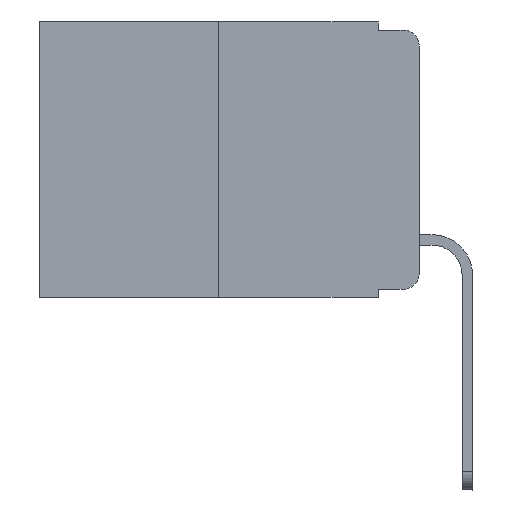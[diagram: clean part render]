
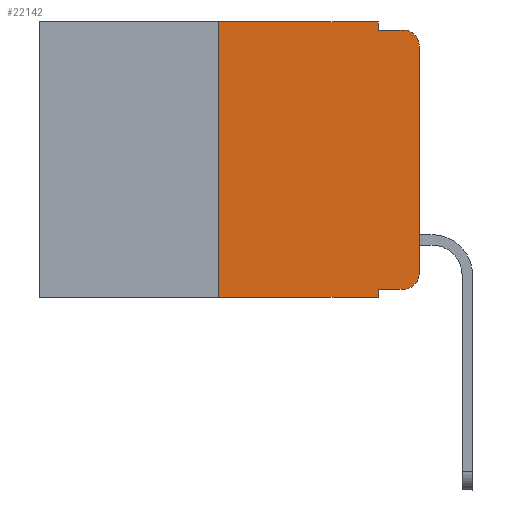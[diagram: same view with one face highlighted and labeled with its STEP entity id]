
A CAD part, left-side view. The second image highlights one B-rep face of the part: STEP entity #22142.
In plain terms, the highlighted planar face has unit normal (-1, 0, 0).
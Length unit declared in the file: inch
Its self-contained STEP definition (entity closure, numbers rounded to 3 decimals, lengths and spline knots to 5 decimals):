
#168 = CARTESIAN_POINT ( 'NONE',  ( 0., 0., -0.313 ) ) ;
#198 = AXIS2_PLACEMENT_3D ( 'NONE', #2361, #24579, #8092 ) ;
#484 = CARTESIAN_POINT ( 'NONE',  ( 0., 0.051, -0.333 ) ) ;
#729 = VERTEX_POINT ( 'NONE', #14420 ) ;
#969 = ORIENTED_EDGE ( 'NONE', *, *, #9742, .T. ) ;
#1007 = LINE ( 'NONE', #8992, #19425 ) ;
#1231 = ORIENTED_EDGE ( 'NONE', *, *, #5311, .F. ) ;
#1653 = ORIENTED_EDGE ( 'NONE', *, *, #17174, .T. ) ;
#1742 = VERTEX_POINT ( 'NONE', #16167 ) ;
#2361 = CARTESIAN_POINT ( 'NONE',  ( 0., 0.02, -0.313 ) ) ;
#2617 = CARTESIAN_POINT ( 'NONE',  ( 0., 0.051, -0.01 ) ) ;
#3530 = CIRCLE ( 'NONE', #18398, 0.02 ) ;
#4014 = ORIENTED_EDGE ( 'NONE', *, *, #21274, .T. ) ;
#4030 = VERTEX_POINT ( 'NONE', #25972 ) ;
#4064 = DIRECTION ( 'NONE',  ( 1., 0., 0. ) ) ;
#4197 = FACE_OUTER_BOUND ( 'NONE', #15719, .T. ) ;
#4251 = VECTOR ( 'NONE', #5102, 39.37008 ) ;
#4290 = CARTESIAN_POINT ( 'NONE',  ( 0., 0.051, -0.333 ) ) ;
#4585 = LINE ( 'NONE', #10703, #9799 ) ;
#4609 = ORIENTED_EDGE ( 'NONE', *, *, #16207, .F. ) ;
#4697 = CARTESIAN_POINT ( 'NONE',  ( 0., 0.02, -0.333 ) ) ;
#5102 = DIRECTION ( 'NONE',  ( 0., 0., 1. ) ) ;
#5311 = EDGE_CURVE ( 'NONE', #1742, #9038, #1007, .T. ) ;
#5446 = LINE ( 'NONE', #19281, #6911 ) ;
#5981 = DIRECTION ( 'NONE',  ( 0., -1., 0. ) ) ;
#6183 = ORIENTED_EDGE ( 'NONE', *, *, #16247, .T. ) ;
#6246 = CARTESIAN_POINT ( 'NONE',  ( 0., 0.02, -0.03 ) ) ;
#6911 = VECTOR ( 'NONE', #5981, 39.37008 ) ;
#7539 = CARTESIAN_POINT ( 'NONE',  ( 0., 0.051, 0. ) ) ;
#8092 = DIRECTION ( 'NONE',  ( 0., 0., -1. ) ) ;
#8992 = CARTESIAN_POINT ( 'NONE',  ( 0., 0.473, 0. ) ) ;
#9038 = VERTEX_POINT ( 'NONE', #22560 ) ;
#9157 = VERTEX_POINT ( 'NONE', #2617 ) ;
#9742 = EDGE_CURVE ( 'NONE', #16116, #15303, #23452, .T. ) ;
#9799 = VECTOR ( 'NONE', #18819, 39.37008 ) ;
#10115 = DIRECTION ( 'NONE',  ( 0., 0., -1. ) ) ;
#10703 = CARTESIAN_POINT ( 'NONE',  ( 0., 0.473, -0.343 ) ) ;
#11433 = CARTESIAN_POINT ( 'NONE',  ( 0., 0.25, 0. ) ) ;
#11484 = CARTESIAN_POINT ( 'NONE',  ( 0., 0., 0. ) ) ;
#12151 = VERTEX_POINT ( 'NONE', #484 ) ;
#12304 = VECTOR ( 'NONE', #13158, 39.37008 ) ;
#12311 = PLANE ( 'NONE',  #19697 ) ;
#13158 = DIRECTION ( 'NONE',  ( 0., -1., 0. ) ) ;
#13243 = DIRECTION ( 'NONE',  ( 0., -1., 0. ) ) ;
#14207 = VECTOR ( 'NONE', #19545, 39.37008 ) ;
#14383 = VERTEX_POINT ( 'NONE', #23779 ) ;
#14413 = DIRECTION ( 'NONE',  ( 0., 0., -1. ) ) ;
#14420 = CARTESIAN_POINT ( 'NONE',  ( 0., 0.25, -0.343 ) ) ;
#14866 = VECTOR ( 'NONE', #14413, 39.37008 ) ;
#15303 = VERTEX_POINT ( 'NONE', #19327 ) ;
#15719 = EDGE_LOOP ( 'NONE', ( #969, #4014, #17935, #16420, #1231, #25223, #1653, #4609, #6183, #16676 ) ) ;
#16116 = VERTEX_POINT ( 'NONE', #168 ) ;
#16167 = CARTESIAN_POINT ( 'NONE',  ( 0., 0.25, 0. ) ) ;
#16207 = EDGE_CURVE ( 'NONE', #12151, #14383, #19401, .T. ) ;
#16247 = EDGE_CURVE ( 'NONE', #12151, #18890, #17296, .T. ) ;
#16420 = ORIENTED_EDGE ( 'NONE', *, *, #16781, .F. ) ;
#16543 = CARTESIAN_POINT ( 'NONE',  ( 0., 0.051, 0. ) ) ;
#16676 = ORIENTED_EDGE ( 'NONE', *, *, #22796, .T. ) ;
#16781 = EDGE_CURVE ( 'NONE', #9038, #9157, #23625, .T. ) ;
#17174 = EDGE_CURVE ( 'NONE', #729, #14383, #4585, .T. ) ;
#17296 = LINE ( 'NONE', #4290, #12304 ) ;
#17935 = ORIENTED_EDGE ( 'NONE', *, *, #19461, .F. ) ;
#18398 = AXIS2_PLACEMENT_3D ( 'NONE', #6246, #20204, #10115 ) ;
#18819 = DIRECTION ( 'NONE',  ( 0., -1., 0. ) ) ;
#18890 = VERTEX_POINT ( 'NONE', #4697 ) ;
#19281 = CARTESIAN_POINT ( 'NONE',  ( 0., 0.051, -0.01 ) ) ;
#19327 = CARTESIAN_POINT ( 'NONE',  ( 0., 0., -0.03 ) ) ;
#19401 = LINE ( 'NONE', #16543, #14866 ) ;
#19425 = VECTOR ( 'NONE', #13243, 39.37008 ) ;
#19461 = EDGE_CURVE ( 'NONE', #9157, #4030, #5446, .T. ) ;
#19545 = DIRECTION ( 'NONE',  ( 0., 0., 1. ) ) ;
#19697 = AXIS2_PLACEMENT_3D ( 'NONE', #20412, #4064, #26147 ) ;
#20204 = DIRECTION ( 'NONE',  ( -1., 0., 0. ) ) ;
#20412 = CARTESIAN_POINT ( 'NONE',  ( 0., 0.473, 0. ) ) ;
#21274 = EDGE_CURVE ( 'NONE', #15303, #4030, #3530, .T. ) ;
#21763 = DIRECTION ( 'NONE',  ( 0., 0., -1. ) ) ;
#22142 = ADVANCED_FACE ( 'NONE', ( #4197 ), #12311, .F. ) ;
#22510 = VECTOR ( 'NONE', #21763, 39.37008 ) ;
#22560 = CARTESIAN_POINT ( 'NONE',  ( 0., 0.051, 0. ) ) ;
#22680 = EDGE_CURVE ( 'NONE', #729, #1742, #25660, .T. ) ;
#22796 = EDGE_CURVE ( 'NONE', #18890, #16116, #23990, .T. ) ;
#23452 = LINE ( 'NONE', #11484, #4251 ) ;
#23625 = LINE ( 'NONE', #7539, #22510 ) ;
#23779 = CARTESIAN_POINT ( 'NONE',  ( 0., 0.051, -0.343 ) ) ;
#23990 = CIRCLE ( 'NONE', #198, 0.02 ) ;
#24579 = DIRECTION ( 'NONE',  ( -1., 0., 0. ) ) ;
#25223 = ORIENTED_EDGE ( 'NONE', *, *, #22680, .F. ) ;
#25660 = LINE ( 'NONE', #11433, #14207 ) ;
#25972 = CARTESIAN_POINT ( 'NONE',  ( 0., 0.02, -0.01 ) ) ;
#26147 = DIRECTION ( 'NONE',  ( 0., 0., -1. ) ) ;
